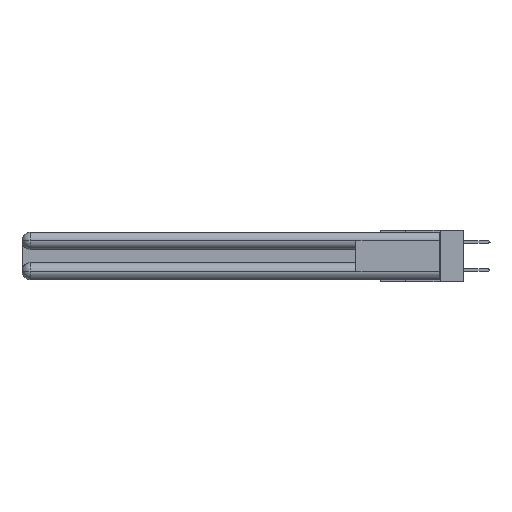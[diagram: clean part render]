
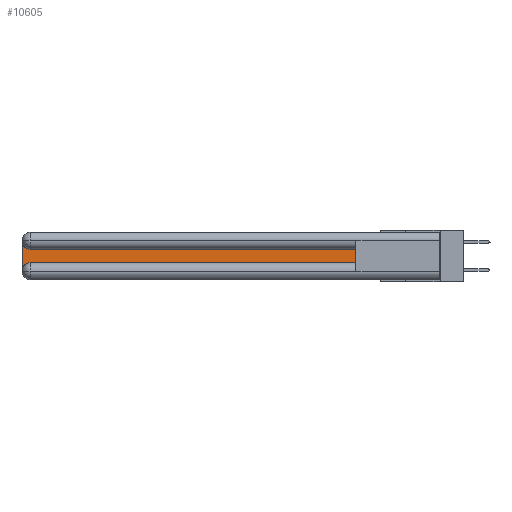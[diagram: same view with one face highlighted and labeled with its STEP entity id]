
A CAD part, left-side view. The second image highlights one B-rep face of the part: STEP entity #10605.
In plain terms, the highlighted planar face has unit normal (-1, 0, 0).
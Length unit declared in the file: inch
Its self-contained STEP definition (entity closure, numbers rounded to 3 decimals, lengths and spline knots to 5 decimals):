
#60 = AXIS2_PLACEMENT_3D ( 'NONE', #21513, #21992, #4405 ) ;
#664 = DIRECTION ( 'NONE',  ( 1., 0., 0. ) ) ;
#717 = ORIENTED_EDGE ( 'NONE', *, *, #10569, .T. ) ;
#848 = CIRCLE ( 'NONE', #60, 0.06 ) ;
#1924 = CARTESIAN_POINT ( 'NONE',  ( 0.075, 0.6, -0.1225 ) ) ;
#2265 = DIRECTION ( 'NONE',  ( 0., -1., 0. ) ) ;
#2305 = EDGE_LOOP ( 'NONE', ( #717, #28439, #15023, #25808, #18175, #6237 ) ) ;
#2321 = EDGE_CURVE ( 'NONE', #12746, #26892, #26296, .T. ) ;
#4085 = EDGE_CURVE ( 'NONE', #9414, #20994, #27605, .T. ) ;
#4405 = DIRECTION ( 'NONE',  ( 0., 0., -1. ) ) ;
#4579 = CARTESIAN_POINT ( 'NONE',  ( 0.075, 3., -0.2175 ) ) ;
#4644 = EDGE_CURVE ( 'NONE', #20994, #7914, #20242, .T. ) ;
#4792 = CARTESIAN_POINT ( 'NONE',  ( 0.075, 0.6, -0.1225 ) ) ;
#5352 = DIRECTION ( 'NONE',  ( 0., 0., -1. ) ) ;
#5900 = DIRECTION ( 'NONE',  ( 0., 0., -1. ) ) ;
#6237 = ORIENTED_EDGE ( 'NONE', *, *, #4644, .T. ) ;
#6752 = CIRCLE ( 'NONE', #17598, 0.06 ) ;
#6987 = EDGE_CURVE ( 'NONE', #12899, #12746, #848, .T. ) ;
#7128 = DIRECTION ( 'NONE',  ( 0., 1., 0. ) ) ;
#7513 = FACE_OUTER_BOUND ( 'NONE', #2305, .T. ) ;
#7726 = CARTESIAN_POINT ( 'NONE',  ( 0.075, 2.94, -0.2175 ) ) ;
#7914 = VERTEX_POINT ( 'NONE', #1924 ) ;
#9235 = CARTESIAN_POINT ( 'NONE',  ( 0.075, 3., -0.2775 ) ) ;
#9414 = VERTEX_POINT ( 'NONE', #7726 ) ;
#10098 = VECTOR ( 'NONE', #20161, 39.37008 ) ;
#10569 = EDGE_CURVE ( 'NONE', #7914, #12899, #14883, .T. ) ;
#10605 = ADVANCED_FACE ( 'NONE', ( #7513 ), #11810, .F. ) ;
#10983 = CARTESIAN_POINT ( 'NONE',  ( 0.075, 0.6, -0.2175 ) ) ;
#11181 = DIRECTION ( 'NONE',  ( 0., 0., -1. ) ) ;
#11810 = PLANE ( 'NONE',  #23394 ) ;
#11911 = CARTESIAN_POINT ( 'NONE',  ( 0.075, 3., -0.1225 ) ) ;
#12746 = VERTEX_POINT ( 'NONE', #20485 ) ;
#12899 = VERTEX_POINT ( 'NONE', #25736 ) ;
#13722 = DIRECTION ( 'NONE',  ( 1., 0., 0. ) ) ;
#14883 = LINE ( 'NONE', #4792, #26091 ) ;
#14981 = CARTESIAN_POINT ( 'NONE',  ( 0.075, 0.6, -0.2175 ) ) ;
#15023 = ORIENTED_EDGE ( 'NONE', *, *, #2321, .T. ) ;
#15417 = VECTOR ( 'NONE', #5900, 39.37008 ) ;
#17598 = AXIS2_PLACEMENT_3D ( 'NONE', #24573, #13722, #11181 ) ;
#18175 = ORIENTED_EDGE ( 'NONE', *, *, #4085, .T. ) ;
#18661 = CARTESIAN_POINT ( 'NONE',  ( 0.075, 0.6, -0.2175 ) ) ;
#20161 = DIRECTION ( 'NONE',  ( 0., 0., 1. ) ) ;
#20242 = LINE ( 'NONE', #14981, #10098 ) ;
#20485 = CARTESIAN_POINT ( 'NONE',  ( 0.075, 3., -0.0625 ) ) ;
#20994 = VERTEX_POINT ( 'NONE', #18661 ) ;
#21513 = CARTESIAN_POINT ( 'NONE',  ( 0.075, 2.94, -0.0625 ) ) ;
#21992 = DIRECTION ( 'NONE',  ( 1., 0., 0. ) ) ;
#23394 = AXIS2_PLACEMENT_3D ( 'NONE', #11911, #664, #5352 ) ;
#24573 = CARTESIAN_POINT ( 'NONE',  ( 0.075, 2.94, -0.2775 ) ) ;
#25736 = CARTESIAN_POINT ( 'NONE',  ( 0.075, 2.94, -0.1225 ) ) ;
#25808 = ORIENTED_EDGE ( 'NONE', *, *, #28577, .T. ) ;
#26091 = VECTOR ( 'NONE', #7128, 39.37008 ) ;
#26296 = LINE ( 'NONE', #4579, #15417 ) ;
#26892 = VERTEX_POINT ( 'NONE', #9235 ) ;
#26898 = VECTOR ( 'NONE', #2265, 39.37008 ) ;
#27605 = LINE ( 'NONE', #10983, #26898 ) ;
#28439 = ORIENTED_EDGE ( 'NONE', *, *, #6987, .T. ) ;
#28577 = EDGE_CURVE ( 'NONE', #26892, #9414, #6752, .T. ) ;
